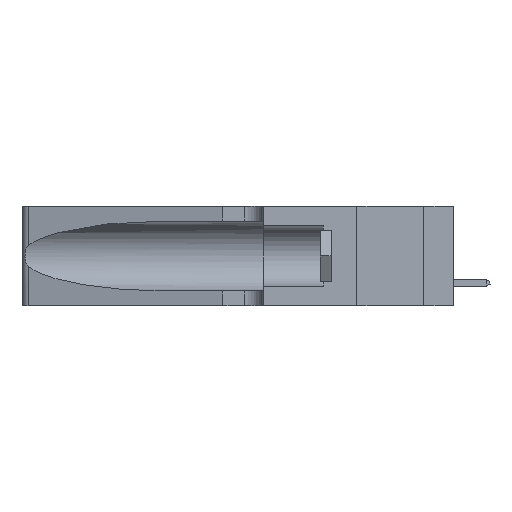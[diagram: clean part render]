
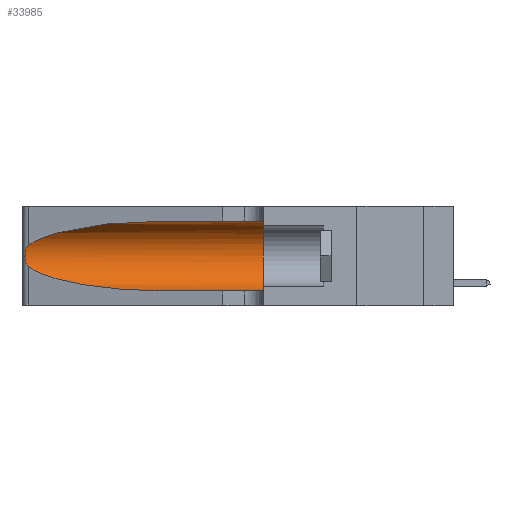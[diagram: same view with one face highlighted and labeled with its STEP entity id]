
A CAD part, left-side view. The second image highlights one B-rep face of the part: STEP entity #33985.
In plain terms, the highlighted cylindrical face has radius 3.308 mm (diameter 6.617 mm), a partial arc.
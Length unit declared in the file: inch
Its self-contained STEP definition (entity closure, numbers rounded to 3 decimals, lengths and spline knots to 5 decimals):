
#625 = DIRECTION ( 'NONE',  ( 0., -1., 0. ) ) ;
#810 = VECTOR ( 'NONE', #29449, 39.37008 ) ;
#941 = CIRCLE ( 'NONE', #8414, 0.13025 ) ;
#1191 = CARTESIAN_POINT ( 'NONE',  ( 0.18966, 0.96281, 0.05475 ) ) ;
#1264 = CARTESIAN_POINT ( 'NONE',  ( 0.25487, 1.22718, 0.14631 ) ) ;
#2552 = DIRECTION ( 'NONE',  ( 0., -1., 0. ) ) ;
#3391 = CARTESIAN_POINT ( 'NONE',  ( 0.1305, 0.72297, 0.05475 ) ) ;
#6164 = CARTESIAN_POINT ( 'NONE',  ( 0.26018, 1.23835, 0.19895 ) ) ;
#8414 = AXIS2_PLACEMENT_3D ( 'NONE', #38303, #46067, #49481 ) ;
#8715 = FACE_OUTER_BOUND ( 'NONE', #37595, .T. ) ;
#8738 = CARTESIAN_POINT ( 'NONE',  ( 0.18966, 0.96281, 0.31525 ) ) ;
#8789 = CARTESIAN_POINT ( 'NONE',  ( 0.2373, 1.15595, 0.08982 ) ) ;
#9407 = CARTESIAN_POINT ( 'NONE',  ( 0.2373, 1.15595, 0.28018 ) ) ;
#9864 = CARTESIAN_POINT ( 'NONE',  ( 0.26075, 1.23896, 0.19203 ) ) ;
#10016 = CARTESIAN_POINT ( 'NONE',  ( 0.1305, 1.61858, 0.31525 ) ) ;
#10923 = ORIENTED_EDGE ( 'NONE', *, *, #40413, .T. ) ;
#13022 = CARTESIAN_POINT ( 'NONE',  ( 0.25487, 1.22718, 0.14631 ) ) ;
#15228 = CARTESIAN_POINT ( 'NONE',  ( 0.1305, 0.35, 0.31525 ) ) ;
#16505 = DIRECTION ( 'NONE',  ( 0., 0., -1. ) ) ;
#16573 = ORIENTED_EDGE ( 'NONE', *, *, #27865, .F. ) ;
#17074 = VECTOR ( 'NONE', #2552, 39.37008 ) ;
#17350 = CARTESIAN_POINT ( 'NONE',  ( 0.1305, 0.35, 0.05475 ) ) ;
#19755 = CARTESIAN_POINT ( 'NONE',  ( 0.25487, 1.22718, 0.22369 ) ) ;
#21134 = CARTESIAN_POINT ( 'NONE',  ( 0.25856, 1.23593, 0.16098 ) ) ;
#21498 = CARTESIAN_POINT ( 'NONE',  ( 0.26075, 1.23896, 0.178 ) ) ;
#21691 = CARTESIAN_POINT ( 'NONE',  ( 0.25487, 1.22718, 0.22369 ) ) ;
#21761 = CARTESIAN_POINT ( 'NONE',  ( 0.25487, 1.22718, 0.22369 ) ) ;
#23485 = VERTEX_POINT ( 'NONE', #29401 ) ;
#24210 = ORIENTED_EDGE ( 'NONE', *, *, #26869, .T. ) ;
#26869 = EDGE_CURVE ( 'NONE', #28916, #27259, #48270, .T. ) ;
#27259 = VERTEX_POINT ( 'NONE', #1264 ) ;
#27536 =( BOUNDED_CURVE ( )  B_SPLINE_CURVE ( 3, ( #27546, #8789, #1191, #27868 ),
 .UNSPECIFIED., .F., .F. ) 
 B_SPLINE_CURVE_WITH_KNOTS ( ( 4, 4 ),
 ( 3.44316, 4.71239 ),
 .UNSPECIFIED. ) 
 CURVE ( )  GEOMETRIC_REPRESENTATION_ITEM ( )  RATIONAL_B_SPLINE_CURVE ( ( 1., 0.87, 0.87, 1. ) ) 
 REPRESENTATION_ITEM ( '' )  );
#27546 = CARTESIAN_POINT ( 'NONE',  ( 0.25487, 1.22718, 0.14631 ) ) ;
#27865 = EDGE_CURVE ( 'NONE', #23485, #29059, #46718, .T. ) ;
#27868 = CARTESIAN_POINT ( 'NONE',  ( 0.1305, 0.72297, 0.05475 ) ) ;
#28916 = VERTEX_POINT ( 'NONE', #19755 ) ;
#29059 = VERTEX_POINT ( 'NONE', #15228 ) ;
#29094 = LINE ( 'NONE', #48936, #17074 ) ;
#29098 = CARTESIAN_POINT ( 'NONE',  ( 0.25789, 1.23486, 0.15765 ) ) ;
#29401 = CARTESIAN_POINT ( 'NONE',  ( 0.1305, 0.72297, 0.31525 ) ) ;
#29449 = DIRECTION ( 'NONE',  ( 0., -1., 0. ) ) ;
#31400 = CARTESIAN_POINT ( 'NONE',  ( 0.25787, 1.23484, 0.2124 ) ) ;
#31578 = VERTEX_POINT ( 'NONE', #3391 ) ;
#32927 = CYLINDRICAL_SURFACE ( 'NONE', #35124, 0.13025 ) ;
#33985 = ADVANCED_FACE ( 'NONE', ( #8715 ), #32927, .F. ) ;
#34757 = EDGE_CURVE ( 'NONE', #23485, #28916, #40845, .T. ) ;
#34893 = ORIENTED_EDGE ( 'NONE', *, *, #47943, .T. ) ;
#35124 = AXIS2_PLACEMENT_3D ( 'NONE', #43448, #625, #16505 ) ;
#36784 = ORIENTED_EDGE ( 'NONE', *, *, #39431, .F. ) ;
#36844 = CARTESIAN_POINT ( 'NONE',  ( 0.26017, 1.23833, 0.17102 ) ) ;
#37595 = EDGE_LOOP ( 'NONE', ( #42043, #24210, #10923, #34893, #36784, #16573 ) ) ;
#38303 = CARTESIAN_POINT ( 'NONE',  ( 0.1305, 0.35, 0.185 ) ) ;
#39431 = EDGE_CURVE ( 'NONE', #29059, #47729, #941, .T. ) ;
#40413 = EDGE_CURVE ( 'NONE', #27259, #31578, #27536, .T. ) ;
#40845 =( BOUNDED_CURVE ( )  B_SPLINE_CURVE ( 3, ( #43971, #8738, #9407, #21761 ),
 .UNSPECIFIED., .F., .F. ) 
 B_SPLINE_CURVE_WITH_KNOTS ( ( 4, 4 ),
 ( 1.5708, 2.84003 ),
 .UNSPECIFIED. ) 
 CURVE ( )  GEOMETRIC_REPRESENTATION_ITEM ( )  RATIONAL_B_SPLINE_CURVE ( ( 1., 0.87, 0.87, 1. ) ) 
 REPRESENTATION_ITEM ( '' )  );
#42043 = ORIENTED_EDGE ( 'NONE', *, *, #34757, .T. ) ;
#43301 = CARTESIAN_POINT ( 'NONE',  ( 0.25639, 1.23184, 0.21858 ) ) ;
#43448 = CARTESIAN_POINT ( 'NONE',  ( 0.1305, 1.61858, 0.185 ) ) ;
#43879 = CARTESIAN_POINT ( 'NONE',  ( 0.25639, 1.23186, 0.15144 ) ) ;
#43971 = CARTESIAN_POINT ( 'NONE',  ( 0.1305, 0.72297, 0.31525 ) ) ;
#46067 = DIRECTION ( 'NONE',  ( 0., 1., 0. ) ) ;
#46718 = LINE ( 'NONE', #10016, #810 ) ;
#47023 = CARTESIAN_POINT ( 'NONE',  ( 0.25555, 1.22994, 0.2215 ) ) ;
#47459 = CARTESIAN_POINT ( 'NONE',  ( 0.25854, 1.2359, 0.20912 ) ) ;
#47729 = VERTEX_POINT ( 'NONE', #17350 ) ;
#47943 = EDGE_CURVE ( 'NONE', #31578, #47729, #29094, .T. ) ;
#48270 = B_SPLINE_CURVE_WITH_KNOTS ( 'NONE', 3,
 ( #21691, #47023, #43301, #31400, #47459, #6164, #9864, #21498, #36844, #21134, #29098, #43879, #48308, #13022 ),
 .UNSPECIFIED., .F., .F.,
 ( 4, 2, 2, 2, 2, 2, 4 ),
 ( 0., 0.00027, 0.00053, 0.00107, 0.0016, 0.00187, 0.00214 ),
 .UNSPECIFIED. ) ;
#48308 = CARTESIAN_POINT ( 'NONE',  ( 0.25555, 1.22993, 0.14849 ) ) ;
#48936 = CARTESIAN_POINT ( 'NONE',  ( 0.1305, 1.61858, 0.05475 ) ) ;
#49481 = DIRECTION ( 'NONE',  ( 0., 0., 1. ) ) ;
